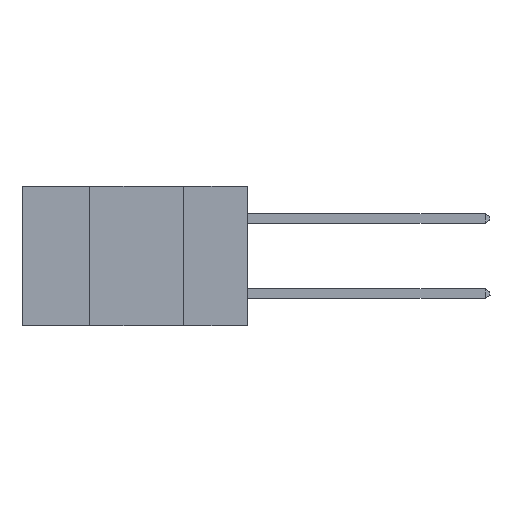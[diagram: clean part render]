
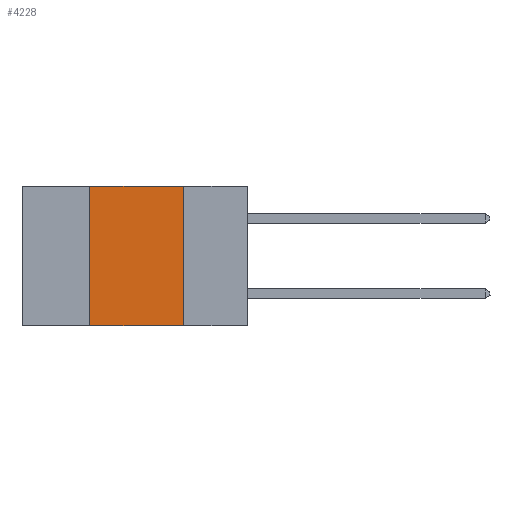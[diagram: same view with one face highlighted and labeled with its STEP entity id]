
A CAD part, left-side view. The second image highlights one B-rep face of the part: STEP entity #4228.
In plain terms, the highlighted planar face has unit normal (-1, 0, 0).
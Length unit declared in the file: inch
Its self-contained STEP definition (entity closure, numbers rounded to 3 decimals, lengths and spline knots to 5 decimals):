
#179 = EDGE_CURVE ( 'NONE', #15392, #13965, #7821, .T. ) ;
#558 = CARTESIAN_POINT ( 'NONE',  ( 0., 0.42, -0.37 ) ) ;
#746 = CARTESIAN_POINT ( 'NONE',  ( 0., 0.17, -0.37 ) ) ;
#760 = DIRECTION ( 'NONE',  ( 0., 0., -1. ) ) ;
#1565 = DIRECTION ( 'NONE',  ( 0., 0., -1. ) ) ;
#2022 = ORIENTED_EDGE ( 'NONE', *, *, #7009, .F. ) ;
#2326 = VECTOR ( 'NONE', #16019, 39.37008 ) ;
#2714 = VECTOR ( 'NONE', #3143, 39.37008 ) ;
#3143 = DIRECTION ( 'NONE',  ( 0., -1., 0. ) ) ;
#3254 = EDGE_LOOP ( 'NONE', ( #6579, #15643, #2022, #11791 ) ) ;
#4066 = VECTOR ( 'NONE', #8165, 39.37008 ) ;
#4228 = ADVANCED_FACE ( 'NONE', ( #10688 ), #14032, .F. ) ;
#4354 = CARTESIAN_POINT ( 'NONE',  ( 0., 0.17, 0. ) ) ;
#5182 = VERTEX_POINT ( 'NONE', #18489 ) ;
#5551 = CARTESIAN_POINT ( 'NONE',  ( 0., 0.42, 0. ) ) ;
#5997 = VERTEX_POINT ( 'NONE', #18024 ) ;
#6579 = ORIENTED_EDGE ( 'NONE', *, *, #13172, .F. ) ;
#7009 = EDGE_CURVE ( 'NONE', #15392, #5997, #18064, .T. ) ;
#7821 = LINE ( 'NONE', #14258, #4066 ) ;
#8165 = DIRECTION ( 'NONE',  ( 0., -1., 0. ) ) ;
#10688 = FACE_OUTER_BOUND ( 'NONE', #3254, .T. ) ;
#11243 = DIRECTION ( 'NONE',  ( 1., 0., 0. ) ) ;
#11791 = ORIENTED_EDGE ( 'NONE', *, *, #179, .T. ) ;
#12033 = CARTESIAN_POINT ( 'NONE',  ( 0., 0.6, 0. ) ) ;
#12476 = LINE ( 'NONE', #12033, #2714 ) ;
#13172 = EDGE_CURVE ( 'NONE', #5182, #13965, #17809, .T. ) ;
#13965 = VERTEX_POINT ( 'NONE', #746 ) ;
#14032 = PLANE ( 'NONE',  #17275 ) ;
#14258 = CARTESIAN_POINT ( 'NONE',  ( 0., 0.6, -0.37 ) ) ;
#14709 = EDGE_CURVE ( 'NONE', #5997, #5182, #12476, .T. ) ;
#15392 = VERTEX_POINT ( 'NONE', #558 ) ;
#15643 = ORIENTED_EDGE ( 'NONE', *, *, #14709, .F. ) ;
#16019 = DIRECTION ( 'NONE',  ( 0., 0., 1. ) ) ;
#17275 = AXIS2_PLACEMENT_3D ( 'NONE', #18563, #11243, #760 ) ;
#17809 = LINE ( 'NONE', #4354, #18061 ) ;
#18024 = CARTESIAN_POINT ( 'NONE',  ( 0., 0.42, 0. ) ) ;
#18061 = VECTOR ( 'NONE', #1565, 39.37008 ) ;
#18064 = LINE ( 'NONE', #5551, #2326 ) ;
#18489 = CARTESIAN_POINT ( 'NONE',  ( 0., 0.17, 0. ) ) ;
#18563 = CARTESIAN_POINT ( 'NONE',  ( 0., 0.6, 0. ) ) ;
